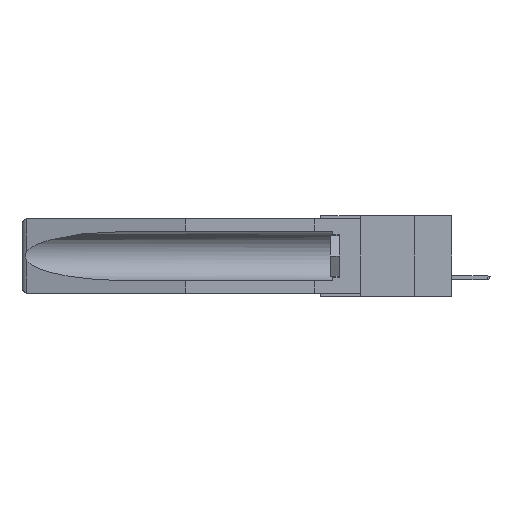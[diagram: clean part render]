
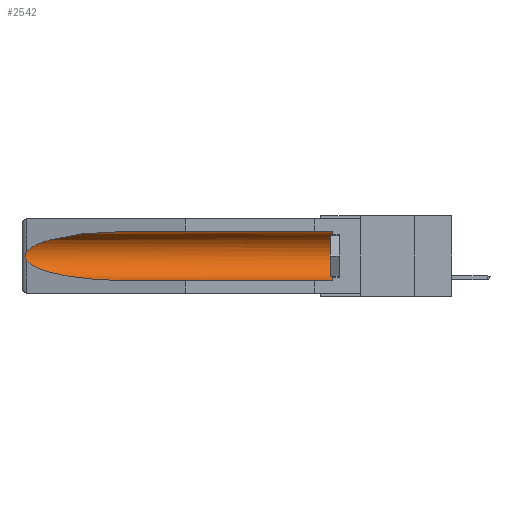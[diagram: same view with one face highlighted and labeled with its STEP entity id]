
A CAD part, left-side view. The second image highlights one B-rep face of the part: STEP entity #2542.
In plain terms, the highlighted cylindrical face has radius 2.857 mm (diameter 5.715 mm), a partial arc.
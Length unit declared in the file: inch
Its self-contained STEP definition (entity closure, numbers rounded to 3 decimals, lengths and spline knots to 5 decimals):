
#225 = EDGE_CURVE ( 'NONE', #1307, #9587, #10745, .T. ) ;
#419 = VECTOR ( 'NONE', #13779, 39.37008 ) ;
#838 = DIRECTION ( 'NONE',  ( 0., 0., 1. ) ) ;
#969 = CARTESIAN_POINT ( 'NONE',  ( 0.25451, 1.48313, -0.24835 ) ) ;
#1307 = VERTEX_POINT ( 'NONE', #5047 ) ;
#1683 = CARTESIAN_POINT ( 'NONE',  ( 0.26654, 1.53092, -0.15636 ) ) ;
#1871 = AXIS2_PLACEMENT_3D ( 'NONE', #14506, #11305, #838 ) ;
#1878 = CARTESIAN_POINT ( 'NONE',  ( 0.26655, 1.53094, -0.18657 ) ) ;
#1925 = AXIS2_PLACEMENT_3D ( 'NONE', #13168, #4251, #2645 ) ;
#2185 = CARTESIAN_POINT ( 'NONE',  ( 0.155, 1.07973, -0.284 ) ) ;
#2436 = VECTOR ( 'NONE', #5970, 39.37008 ) ;
#2542 = ADVANCED_FACE ( 'NONE', ( #4087 ), #5034, .F. ) ;
#2645 = DIRECTION ( 'NONE',  ( 0., 0., 1. ) ) ;
#2850 = ORIENTED_EDGE ( 'NONE', *, *, #18350, .T. ) ;
#2914 = ORIENTED_EDGE ( 'NONE', *, *, #17885, .F. ) ;
#3343 = EDGE_CURVE ( 'NONE', #5394, #1307, #19050, .T. ) ;
#3716 = ORIENTED_EDGE ( 'NONE', *, *, #225, .T. ) ;
#4087 = FACE_OUTER_BOUND ( 'NONE', #6127, .T. ) ;
#4251 = DIRECTION ( 'NONE',  ( 0., -1., 0. ) ) ;
#4889 = CARTESIAN_POINT ( 'NONE',  ( 0.2675, 1.53308, -0.16763 ) ) ;
#5030 = CARTESIAN_POINT ( 'NONE',  ( 0.2673, 1.5327, -0.16383 ) ) ;
#5034 = CYLINDRICAL_SURFACE ( 'NONE', #1871, 0.1125 ) ;
#5047 = CARTESIAN_POINT ( 'NONE',  ( 0.155, 1.07973, -0.059 ) ) ;
#5394 = VERTEX_POINT ( 'NONE', #15068 ) ;
#5612 = CARTESIAN_POINT ( 'NONE',  ( 0.26537, 1.52718, -0.14972 ) ) ;
#5703 = ORIENTED_EDGE ( 'NONE', *, *, #3343, .T. ) ;
#5970 = DIRECTION ( 'NONE',  ( 0., 1., 0. ) ) ;
#6092 = CARTESIAN_POINT ( 'NONE',  ( 0.155, -0.30754, -0.284 ) ) ;
#6127 = EDGE_LOOP ( 'NONE', ( #3716, #12210, #2850, #2914, #13468, #5703 ) ) ;
#6292 = CARTESIAN_POINT ( 'NONE',  ( 0.26597, 1.5296, -0.19026 ) ) ;
#6549 = CARTESIAN_POINT ( 'NONE',  ( 0.26537, 1.52718, -0.19328 ) ) ;
#6764 = CARTESIAN_POINT ( 'NONE',  ( 0.26537, 1.52718, -0.14972 ) ) ;
#7187 = CARTESIAN_POINT ( 'NONE',  ( 0.26537, 1.52718, -0.19328 ) ) ;
#8167 = CARTESIAN_POINT ( 'NONE',  ( 0.155, 1.07973, -0.059 ) ) ;
#8413 = CARTESIAN_POINT ( 'NONE',  ( 0.21114, 1.30732, -0.059 ) ) ;
#8690 = CARTESIAN_POINT ( 'NONE',  ( 0.21114, 1.30732, -0.284 ) ) ;
#8857 = EDGE_CURVE ( 'NONE', #9587, #11437, #14294, .T. ) ;
#9326 = CARTESIAN_POINT ( 'NONE',  ( 0.155, -0.30754, -0.059 ) ) ;
#9366 = CARTESIAN_POINT ( 'NONE',  ( 0.155, 0.126, -0.284 ) ) ;
#9540 = CARTESIAN_POINT ( 'NONE',  ( 0.26537, 1.52718, -0.14972 ) ) ;
#9587 = VERTEX_POINT ( 'NONE', #5612 ) ;
#9887 =( BOUNDED_CURVE ( )  B_SPLINE_CURVE ( 3, ( #7187, #969, #8690, #13238 ),
 .UNSPECIFIED., .F., .F. ) 
 B_SPLINE_CURVE_WITH_KNOTS ( ( 4, 4 ),
 ( 0.1948, 1.5708 ),
 .UNSPECIFIED. ) 
 CURVE ( )  GEOMETRIC_REPRESENTATION_ITEM ( )  RATIONAL_B_SPLINE_CURVE ( ( 1., 0.848, 0.848, 1. ) ) 
 REPRESENTATION_ITEM ( '' )  );
#10018 = VERTEX_POINT ( 'NONE', #9366 ) ;
#10527 = LINE ( 'NONE', #6092, #2436 ) ;
#10686 = VERTEX_POINT ( 'NONE', #2185 ) ;
#10745 =( BOUNDED_CURVE ( )  B_SPLINE_CURVE ( 3, ( #8167, #8413, #15949, #6764 ),
 .UNSPECIFIED., .F., .F. ) 
 B_SPLINE_CURVE_WITH_KNOTS ( ( 4, 4 ),
 ( 4.71239, 6.08839 ),
 .UNSPECIFIED. ) 
 CURVE ( )  GEOMETRIC_REPRESENTATION_ITEM ( )  RATIONAL_B_SPLINE_CURVE ( ( 1., 0.848, 0.848, 1. ) ) 
 REPRESENTATION_ITEM ( '' )  );
#10800 = CIRCLE ( 'NONE', #1925, 0.1125 ) ;
#10936 = CARTESIAN_POINT ( 'NONE',  ( 0.2673, 1.53269, -0.17917 ) ) ;
#11002 = CARTESIAN_POINT ( 'NONE',  ( 0.26597, 1.52961, -0.15275 ) ) ;
#11305 = DIRECTION ( 'NONE',  ( 0., 1., 0. ) ) ;
#11437 = VERTEX_POINT ( 'NONE', #18504 ) ;
#12210 = ORIENTED_EDGE ( 'NONE', *, *, #8857, .T. ) ;
#13168 = CARTESIAN_POINT ( 'NONE',  ( 0.155, 0.126, -0.1715 ) ) ;
#13238 = CARTESIAN_POINT ( 'NONE',  ( 0.155, 1.07973, -0.284 ) ) ;
#13468 = ORIENTED_EDGE ( 'NONE', *, *, #17268, .T. ) ;
#13779 = DIRECTION ( 'NONE',  ( 0., 1., 0. ) ) ;
#13932 = CARTESIAN_POINT ( 'NONE',  ( 0.2675, 1.53308, -0.17534 ) ) ;
#14294 = B_SPLINE_CURVE_WITH_KNOTS ( 'NONE', 3,
 ( #9540, #11002, #1683, #5030, #4889, #13932, #10936, #1878, #6292, #6549 ),
 .UNSPECIFIED., .F., .F.,
 ( 4, 2, 2, 2, 4 ),
 ( 0., 0.00029, 0.00058, 0.00087, 0.00117 ),
 .UNSPECIFIED. ) ;
#14506 = CARTESIAN_POINT ( 'NONE',  ( 0.155, -0.30754, -0.1715 ) ) ;
#15068 = CARTESIAN_POINT ( 'NONE',  ( 0.155, 0.126, -0.059 ) ) ;
#15949 = CARTESIAN_POINT ( 'NONE',  ( 0.25451, 1.48313, -0.09465 ) ) ;
#17268 = EDGE_CURVE ( 'NONE', #10018, #5394, #10800, .T. ) ;
#17885 = EDGE_CURVE ( 'NONE', #10018, #10686, #10527, .T. ) ;
#18350 = EDGE_CURVE ( 'NONE', #11437, #10686, #9887, .T. ) ;
#18504 = CARTESIAN_POINT ( 'NONE',  ( 0.26537, 1.52718, -0.19328 ) ) ;
#19050 = LINE ( 'NONE', #9326, #419 ) ;
